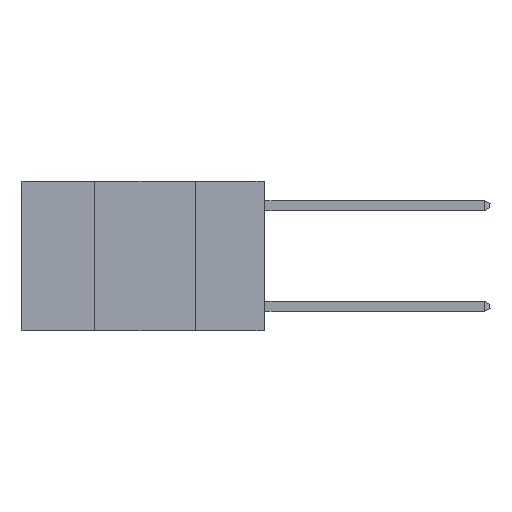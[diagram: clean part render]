
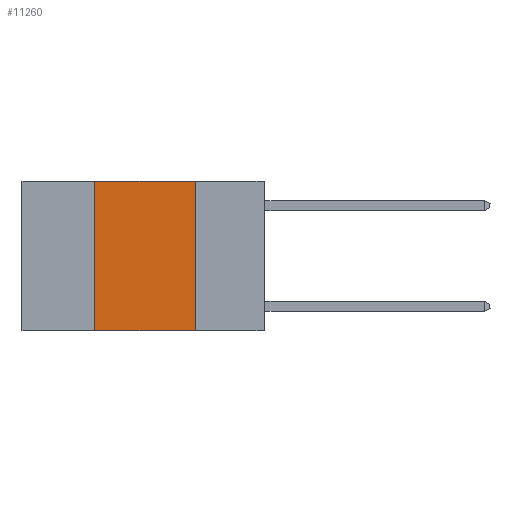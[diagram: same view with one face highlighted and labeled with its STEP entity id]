
A CAD part, left-side view. The second image highlights one B-rep face of the part: STEP entity #11260.
In plain terms, the highlighted planar face has unit normal (-1, 0, 0).
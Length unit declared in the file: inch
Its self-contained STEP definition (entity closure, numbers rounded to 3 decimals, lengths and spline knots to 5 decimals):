
#885 = AXIS2_PLACEMENT_3D ( 'NONE', #25477, #11900, #25862 ) ;
#1501 = VECTOR ( 'NONE', #21791, 39.37008 ) ;
#1764 = EDGE_LOOP ( 'NONE', ( #23544, #4057, #14330, #5810 ) ) ;
#2575 = EDGE_CURVE ( 'NONE', #7337, #15623, #2596, .T. ) ;
#2596 = LINE ( 'NONE', #13209, #1501 ) ;
#4057 = ORIENTED_EDGE ( 'NONE', *, *, #15571, .F. ) ;
#4846 = VECTOR ( 'NONE', #12655, 39.37008 ) ;
#5369 = CARTESIAN_POINT ( 'NONE',  ( 0., 0.17, 0. ) ) ;
#5810 = ORIENTED_EDGE ( 'NONE', *, *, #23740, .T. ) ;
#7180 = VECTOR ( 'NONE', #16579, 39.37008 ) ;
#7337 = VERTEX_POINT ( 'NONE', #5369 ) ;
#7458 = LINE ( 'NONE', #15495, #14837 ) ;
#7864 = DIRECTION ( 'NONE',  ( 0., -1., 0. ) ) ;
#10507 = CARTESIAN_POINT ( 'NONE',  ( 0., 0.6, -0.37 ) ) ;
#10545 = CARTESIAN_POINT ( 'NONE',  ( 0., 0.42, 0. ) ) ;
#11260 = ADVANCED_FACE ( 'NONE', ( #11362 ), #25737, .F. ) ;
#11362 = FACE_OUTER_BOUND ( 'NONE', #1764, .T. ) ;
#11900 = DIRECTION ( 'NONE',  ( 1., 0., 0. ) ) ;
#12655 = DIRECTION ( 'NONE',  ( 0., 0., 1. ) ) ;
#13209 = CARTESIAN_POINT ( 'NONE',  ( 0., 0.17, 0. ) ) ;
#14207 = VERTEX_POINT ( 'NONE', #18010 ) ;
#14330 = ORIENTED_EDGE ( 'NONE', *, *, #17537, .F. ) ;
#14837 = VECTOR ( 'NONE', #7864, 39.37008 ) ;
#15495 = CARTESIAN_POINT ( 'NONE',  ( 0., 0.6, 0. ) ) ;
#15571 = EDGE_CURVE ( 'NONE', #15602, #7337, #7458, .T. ) ;
#15602 = VERTEX_POINT ( 'NONE', #24158 ) ;
#15623 = VERTEX_POINT ( 'NONE', #20083 ) ;
#16579 = DIRECTION ( 'NONE',  ( 0., -1., 0. ) ) ;
#17537 = EDGE_CURVE ( 'NONE', #14207, #15602, #22392, .T. ) ;
#18010 = CARTESIAN_POINT ( 'NONE',  ( 0., 0.42, -0.37 ) ) ;
#18554 = LINE ( 'NONE', #10507, #7180 ) ;
#20083 = CARTESIAN_POINT ( 'NONE',  ( 0., 0.17, -0.37 ) ) ;
#21791 = DIRECTION ( 'NONE',  ( 0., 0., -1. ) ) ;
#22392 = LINE ( 'NONE', #10545, #4846 ) ;
#23544 = ORIENTED_EDGE ( 'NONE', *, *, #2575, .F. ) ;
#23740 = EDGE_CURVE ( 'NONE', #14207, #15623, #18554, .T. ) ;
#24158 = CARTESIAN_POINT ( 'NONE',  ( 0., 0.42, 0. ) ) ;
#25477 = CARTESIAN_POINT ( 'NONE',  ( 0., 0.6, 0. ) ) ;
#25737 = PLANE ( 'NONE',  #885 ) ;
#25862 = DIRECTION ( 'NONE',  ( 0., 0., -1. ) ) ;
